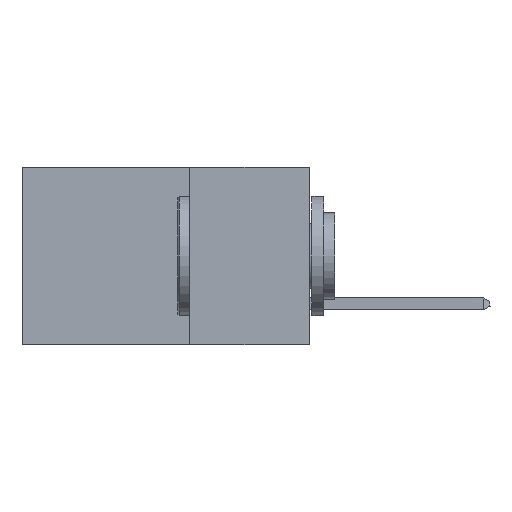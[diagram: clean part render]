
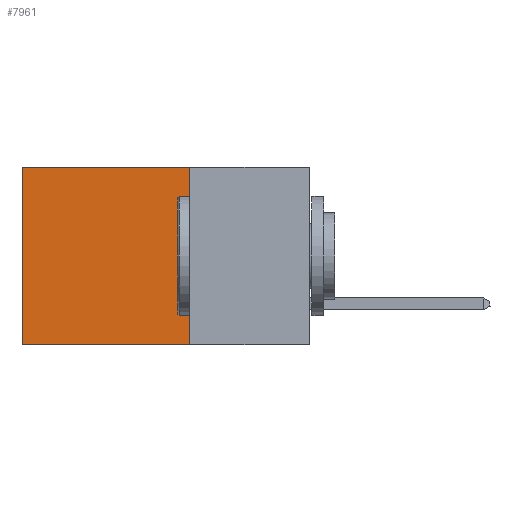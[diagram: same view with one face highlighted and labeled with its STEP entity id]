
A CAD part, left-side view. The second image highlights one B-rep face of the part: STEP entity #7961.
In plain terms, the highlighted planar face has unit normal (-1, 0, 0).
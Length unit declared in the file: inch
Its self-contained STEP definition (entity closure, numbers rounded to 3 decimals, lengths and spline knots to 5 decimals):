
#241 = LINE ( 'NONE', #14985, #3244 ) ;
#883 = VERTEX_POINT ( 'NONE', #16670 ) ;
#1747 = ORIENTED_EDGE ( 'NONE', *, *, #23416, .F. ) ;
#3131 = VERTEX_POINT ( 'NONE', #18804 ) ;
#3244 = VECTOR ( 'NONE', #19911, 39.37008 ) ;
#4050 = FACE_OUTER_BOUND ( 'NONE', #20081, .T. ) ;
#4627 = VERTEX_POINT ( 'NONE', #14549 ) ;
#6641 = DIRECTION ( 'NONE',  ( 0., 1., 0. ) ) ;
#7961 = ADVANCED_FACE ( 'NONE', ( #4050 ), #28226, .F. ) ;
#8330 = LINE ( 'NONE', #11549, #19555 ) ;
#9340 = CARTESIAN_POINT ( 'NONE',  ( 0.2875, 0.25, 0. ) ) ;
#11205 = CARTESIAN_POINT ( 'NONE',  ( 0.2875, 0.6, 0. ) ) ;
#11239 = CARTESIAN_POINT ( 'NONE',  ( 0.2875, 0.25, 0. ) ) ;
#11549 = CARTESIAN_POINT ( 'NONE',  ( 0.2875, 0.25, -0.37 ) ) ;
#11622 = ORIENTED_EDGE ( 'NONE', *, *, #24204, .T. ) ;
#11845 = DIRECTION ( 'NONE',  ( 0., 0., -1. ) ) ;
#12143 = EDGE_CURVE ( 'NONE', #3131, #883, #241, .T. ) ;
#12368 = VECTOR ( 'NONE', #19882, 39.37008 ) ;
#12630 = VECTOR ( 'NONE', #20718, 39.37008 ) ;
#14549 = CARTESIAN_POINT ( 'NONE',  ( 0.2875, 0.6, 0. ) ) ;
#14561 = ORIENTED_EDGE ( 'NONE', *, *, #12143, .F. ) ;
#14985 = CARTESIAN_POINT ( 'NONE',  ( 0.2875, 0.25, 0. ) ) ;
#14992 = CARTESIAN_POINT ( 'NONE',  ( 0.2875, 0.6, -0.37 ) ) ;
#16670 = CARTESIAN_POINT ( 'NONE',  ( 0.2875, 0.25, -0.37 ) ) ;
#17900 = LINE ( 'NONE', #11205, #12630 ) ;
#18804 = CARTESIAN_POINT ( 'NONE',  ( 0.2875, 0.25, 0. ) ) ;
#18917 = ORIENTED_EDGE ( 'NONE', *, *, #29195, .T. ) ;
#19555 = VECTOR ( 'NONE', #6641, 39.37008 ) ;
#19882 = DIRECTION ( 'NONE',  ( 0., 1., 0. ) ) ;
#19911 = DIRECTION ( 'NONE',  ( 0., 0., -1. ) ) ;
#20081 = EDGE_LOOP ( 'NONE', ( #18917, #1747, #14561, #11622 ) ) ;
#20718 = DIRECTION ( 'NONE',  ( 0., 0., -1. ) ) ;
#23416 = EDGE_CURVE ( 'NONE', #883, #29133, #8330, .T. ) ;
#24204 = EDGE_CURVE ( 'NONE', #3131, #4627, #28900, .T. ) ;
#26151 = DIRECTION ( 'NONE',  ( 1., 0., 0. ) ) ;
#26480 = AXIS2_PLACEMENT_3D ( 'NONE', #11239, #26151, #11845 ) ;
#28226 = PLANE ( 'NONE',  #26480 ) ;
#28900 = LINE ( 'NONE', #9340, #12368 ) ;
#29133 = VERTEX_POINT ( 'NONE', #14992 ) ;
#29195 = EDGE_CURVE ( 'NONE', #4627, #29133, #17900, .T. ) ;
